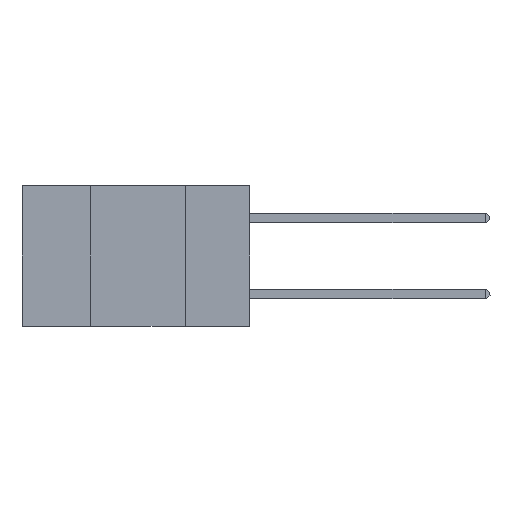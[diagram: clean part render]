
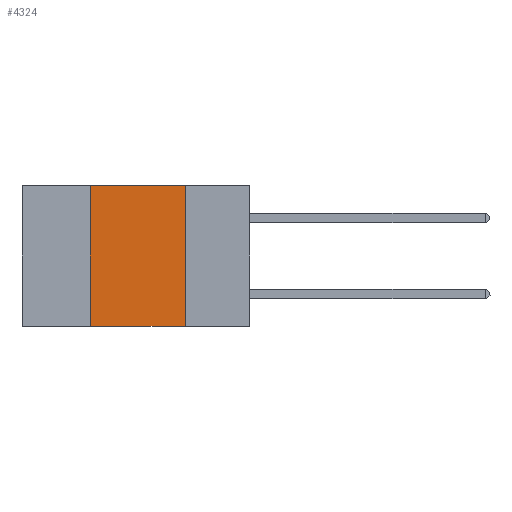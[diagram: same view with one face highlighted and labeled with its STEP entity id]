
A CAD part, left-side view. The second image highlights one B-rep face of the part: STEP entity #4324.
In plain terms, the highlighted planar face has unit normal (-1, 0, 0).
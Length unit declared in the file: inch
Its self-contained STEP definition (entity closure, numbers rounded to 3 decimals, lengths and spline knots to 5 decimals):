
#360 = CARTESIAN_POINT ( 'NONE',  ( 0., 0.17, 0. ) ) ;
#1090 = ORIENTED_EDGE ( 'NONE', *, *, #2501, .F. ) ;
#1638 = CARTESIAN_POINT ( 'NONE',  ( 0., 0.42, 0. ) ) ;
#2019 = PLANE ( 'NONE',  #13727 ) ;
#2046 = VERTEX_POINT ( 'NONE', #8737 ) ;
#2071 = CARTESIAN_POINT ( 'NONE',  ( 0., 0.6, -0.37 ) ) ;
#2352 = DIRECTION ( 'NONE',  ( 0., 0., -1. ) ) ;
#2501 = EDGE_CURVE ( 'NONE', #11335, #9383, #11302, .T. ) ;
#2898 = EDGE_CURVE ( 'NONE', #9383, #9581, #5828, .T. ) ;
#3086 = LINE ( 'NONE', #360, #3240 ) ;
#3238 = ORIENTED_EDGE ( 'NONE', *, *, #4291, .T. ) ;
#3240 = VECTOR ( 'NONE', #2352, 39.37008 ) ;
#3877 = CARTESIAN_POINT ( 'NONE',  ( 0., 0.42, 0. ) ) ;
#4100 = FACE_OUTER_BOUND ( 'NONE', #5998, .T. ) ;
#4291 = EDGE_CURVE ( 'NONE', #11335, #2046, #11608, .T. ) ;
#4324 = ADVANCED_FACE ( 'NONE', ( #4100 ), #2019, .F. ) ;
#5828 = LINE ( 'NONE', #5937, #13556 ) ;
#5937 = CARTESIAN_POINT ( 'NONE',  ( 0., 0.6, 0. ) ) ;
#5998 = EDGE_LOOP ( 'NONE', ( #6129, #10373, #1090, #3238 ) ) ;
#6129 = ORIENTED_EDGE ( 'NONE', *, *, #9615, .F. ) ;
#6308 = VECTOR ( 'NONE', #12763, 39.37008 ) ;
#6366 = VECTOR ( 'NONE', #11407, 39.37008 ) ;
#7268 = CARTESIAN_POINT ( 'NONE',  ( 0., 0.42, -0.37 ) ) ;
#8583 = CARTESIAN_POINT ( 'NONE',  ( 0., 0.17, 0. ) ) ;
#8737 = CARTESIAN_POINT ( 'NONE',  ( 0., 0.17, -0.37 ) ) ;
#9383 = VERTEX_POINT ( 'NONE', #1638 ) ;
#9581 = VERTEX_POINT ( 'NONE', #8583 ) ;
#9615 = EDGE_CURVE ( 'NONE', #9581, #2046, #3086, .T. ) ;
#10373 = ORIENTED_EDGE ( 'NONE', *, *, #2898, .F. ) ;
#11302 = LINE ( 'NONE', #3877, #6366 ) ;
#11335 = VERTEX_POINT ( 'NONE', #7268 ) ;
#11407 = DIRECTION ( 'NONE',  ( 0., 0., 1. ) ) ;
#11608 = LINE ( 'NONE', #2071, #6308 ) ;
#12763 = DIRECTION ( 'NONE',  ( 0., -1., 0. ) ) ;
#12809 = CARTESIAN_POINT ( 'NONE',  ( 0., 0.6, 0. ) ) ;
#13556 = VECTOR ( 'NONE', #13801, 39.37008 ) ;
#13727 = AXIS2_PLACEMENT_3D ( 'NONE', #12809, #14065, #14107 ) ;
#13801 = DIRECTION ( 'NONE',  ( 0., -1., 0. ) ) ;
#14065 = DIRECTION ( 'NONE',  ( 1., 0., 0. ) ) ;
#14107 = DIRECTION ( 'NONE',  ( 0., 0., -1. ) ) ;
